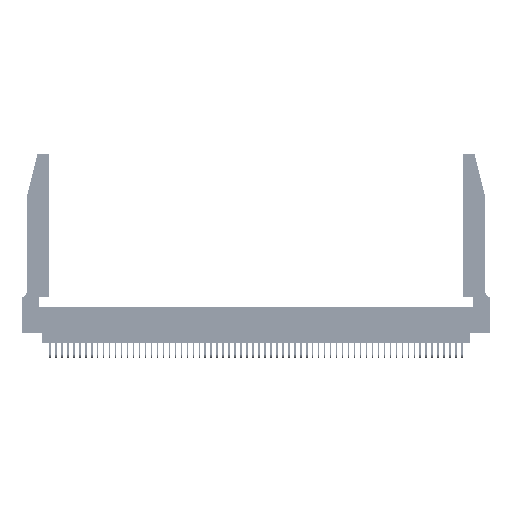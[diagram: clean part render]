
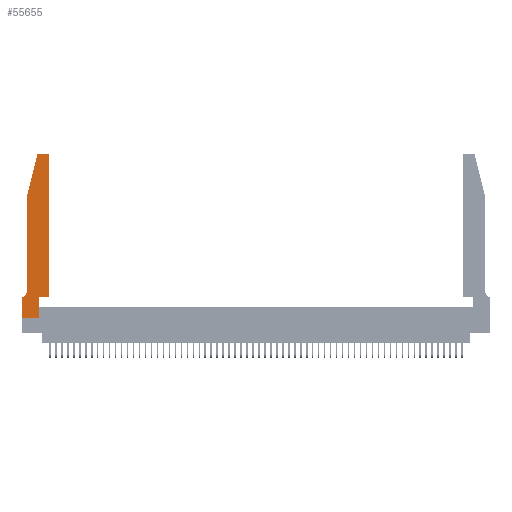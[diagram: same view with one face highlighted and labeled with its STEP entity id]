
A CAD part, top view. The second image highlights one B-rep face of the part: STEP entity #55655.
In plain terms, the highlighted planar face has unit normal (0, 0, 1).
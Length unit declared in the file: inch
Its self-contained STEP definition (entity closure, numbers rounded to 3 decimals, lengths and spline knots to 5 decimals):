
#858 = LINE ( 'NONE', #16642, #51080 ) ;
#1487 = VERTEX_POINT ( 'NONE', #41940 ) ;
#1556 = ORIENTED_EDGE ( 'NONE', *, *, #45499, .T. ) ;
#1739 = CARTESIAN_POINT ( 'NONE',  ( 0.2605, 2.75, 0.37 ) ) ;
#2333 = DIRECTION ( 'NONE',  ( 1., 0., 0. ) ) ;
#2833 = DIRECTION ( 'NONE',  ( 1., 0., 0. ) ) ;
#4481 = DIRECTION ( 'NONE',  ( 0., 0., 1. ) ) ;
#5484 = VERTEX_POINT ( 'NONE', #19264 ) ;
#6705 = CARTESIAN_POINT ( 'NONE',  ( 0.0755, 2., 0.37 ) ) ;
#7498 = ORIENTED_EDGE ( 'NONE', *, *, #34452, .T. ) ;
#7629 = VERTEX_POINT ( 'NONE', #12851 ) ;
#7697 = DIRECTION ( 'NONE',  ( 1., 0., 0. ) ) ;
#7972 = CARTESIAN_POINT ( 'NONE',  ( 0.0755, 0.35, 0.37 ) ) ;
#8842 = LINE ( 'NONE', #7972, #43009 ) ;
#9622 = CARTESIAN_POINT ( 'NONE',  ( 0.4205, 2.75, 0.37 ) ) ;
#10423 = AXIS2_PLACEMENT_3D ( 'NONE', #27438, #49858, #31884 ) ;
#10427 = AXIS2_PLACEMENT_3D ( 'NONE', #14665, #54387, #36827 ) ;
#10668 = AXIS2_PLACEMENT_3D ( 'NONE', #55692, #56073, #2333 ) ;
#10901 = FACE_OUTER_BOUND ( 'NONE', #43075, .T. ) ;
#11278 = DIRECTION ( 'NONE',  ( -1., 0., 0. ) ) ;
#11586 = DIRECTION ( 'NONE',  ( -0.239, -0.971, 0. ) ) ;
#11869 = CARTESIAN_POINT ( 'NONE',  ( 0.2865, 0.35, 0.37 ) ) ;
#12851 = CARTESIAN_POINT ( 'NONE',  ( 0.284, 2.75, 0.37 ) ) ;
#13425 = DIRECTION ( 'NONE',  ( 1., 0., 0. ) ) ;
#13940 = VECTOR ( 'NONE', #46292, 39.37008 ) ;
#14355 = ORIENTED_EDGE ( 'NONE', *, *, #27816, .T. ) ;
#14366 = LINE ( 'NONE', #51479, #42988 ) ;
#14377 = VECTOR ( 'NONE', #28451, 39.37008 ) ;
#14665 = CARTESIAN_POINT ( 'NONE',  ( 0.0055, 0.42, 0.37 ) ) ;
#14832 = CARTESIAN_POINT ( 'NONE',  ( 0.0755, 0.42, 0.37 ) ) ;
#16642 = CARTESIAN_POINT ( 'NONE',  ( 0., 0., 0.37 ) ) ;
#16815 = CARTESIAN_POINT ( 'NONE',  ( 0.4505, 0.35, 0.37 ) ) ;
#16957 = VERTEX_POINT ( 'NONE', #27746 ) ;
#17248 = ORIENTED_EDGE ( 'NONE', *, *, #18725, .T. ) ;
#18233 = EDGE_CURVE ( 'NONE', #22236, #16957, #29174, .T. ) ;
#18445 = EDGE_CURVE ( 'NONE', #31850, #26766, #36559, .T. ) ;
#18725 = EDGE_CURVE ( 'NONE', #16957, #31850, #8842, .T. ) ;
#18949 = LINE ( 'NONE', #29277, #37075 ) ;
#19264 = CARTESIAN_POINT ( 'NONE',  ( 0.25487, 2.72718, 0.37 ) ) ;
#20442 = VERTEX_POINT ( 'NONE', #11869 ) ;
#21576 = CARTESIAN_POINT ( 'NONE',  ( 0.4205, 2.72, 0.37 ) ) ;
#22236 = VERTEX_POINT ( 'NONE', #14832 ) ;
#22560 = CIRCLE ( 'NONE', #24779, 0.03 ) ;
#22872 = CARTESIAN_POINT ( 'NONE',  ( 0., 0., 0.37 ) ) ;
#24610 = VECTOR ( 'NONE', #11278, 39.37008 ) ;
#24753 = DIRECTION ( 'NONE',  ( 0., 1., 0. ) ) ;
#24779 = AXIS2_PLACEMENT_3D ( 'NONE', #21576, #4481, #13425 ) ;
#25440 = VERTEX_POINT ( 'NONE', #9622 ) ;
#25699 = EDGE_CURVE ( 'NONE', #1487, #20442, #14366, .T. ) ;
#26766 = VERTEX_POINT ( 'NONE', #22872 ) ;
#27021 = ORIENTED_EDGE ( 'NONE', *, *, #29974, .T. ) ;
#27438 = CARTESIAN_POINT ( 'NONE',  ( 0., 0.35, 0.37 ) ) ;
#27746 = CARTESIAN_POINT ( 'NONE',  ( 0.0055, 0.35, 0.37 ) ) ;
#27816 = EDGE_CURVE ( 'NONE', #28068, #25440, #22560, .T. ) ;
#28068 = VERTEX_POINT ( 'NONE', #37316 ) ;
#28074 = LINE ( 'NONE', #29671, #30833 ) ;
#28451 = DIRECTION ( 'NONE',  ( 0., -1., 0. ) ) ;
#28701 = CARTESIAN_POINT ( 'NONE',  ( 0.0755, 2., 0.37 ) ) ;
#29174 = CIRCLE ( 'NONE', #10427, 0.07 ) ;
#29277 = CARTESIAN_POINT ( 'NONE',  ( 0.0755, 2., 0.37 ) ) ;
#29671 = CARTESIAN_POINT ( 'NONE',  ( 0.4505, 0.35, 0.37 ) ) ;
#29974 = EDGE_CURVE ( 'NONE', #51574, #22236, #39682, .T. ) ;
#30833 = VECTOR ( 'NONE', #2833, 39.37008 ) ;
#31828 = CARTESIAN_POINT ( 'NONE',  ( 0., 0.35, 0.37 ) ) ;
#31850 = VERTEX_POINT ( 'NONE', #31828 ) ;
#31884 = DIRECTION ( 'NONE',  ( 1., 0., 0. ) ) ;
#31935 = CARTESIAN_POINT ( 'NONE',  ( 0.4505, 0.35, 0.37 ) ) ;
#32760 = CARTESIAN_POINT ( 'NONE',  ( 0., 0., 0.37 ) ) ;
#32862 = ORIENTED_EDGE ( 'NONE', *, *, #35316, .T. ) ;
#34040 = ORIENTED_EDGE ( 'NONE', *, *, #18445, .T. ) ;
#34452 = EDGE_CURVE ( 'NONE', #25440, #7629, #53190, .T. ) ;
#34831 = DIRECTION ( 'NONE',  ( -1., 0., 0. ) ) ;
#35316 = EDGE_CURVE ( 'NONE', #5484, #51574, #18949, .T. ) ;
#36559 = LINE ( 'NONE', #32760, #14377 ) ;
#36784 = LINE ( 'NONE', #31935, #43815 ) ;
#36827 = DIRECTION ( 'NONE',  ( -1., 0., 0. ) ) ;
#37075 = VECTOR ( 'NONE', #11586, 39.37008 ) ;
#37316 = CARTESIAN_POINT ( 'NONE',  ( 0.4505, 2.72, 0.37 ) ) ;
#38027 = EDGE_CURVE ( 'NONE', #20442, #43602, #28074, .T. ) ;
#38646 = EDGE_CURVE ( 'NONE', #26766, #1487, #858, .T. ) ;
#39682 = LINE ( 'NONE', #28701, #13940 ) ;
#39972 = EDGE_CURVE ( 'NONE', #7629, #5484, #48799, .T. ) ;
#41940 = CARTESIAN_POINT ( 'NONE',  ( 0.2865, 0., 0.37 ) ) ;
#42988 = VECTOR ( 'NONE', #24753, 39.37008 ) ;
#43009 = VECTOR ( 'NONE', #34831, 39.37008 ) ;
#43075 = EDGE_LOOP ( 'NONE', ( #7498, #53590, #32862, #27021, #45960, #17248, #34040, #44495, #45604, #52550, #1556, #14355 ) ) ;
#43602 = VERTEX_POINT ( 'NONE', #16815 ) ;
#43815 = VECTOR ( 'NONE', #45235, 39.37008 ) ;
#44495 = ORIENTED_EDGE ( 'NONE', *, *, #38646, .T. ) ;
#45235 = DIRECTION ( 'NONE',  ( 0., 1., 0. ) ) ;
#45499 = EDGE_CURVE ( 'NONE', #43602, #28068, #36784, .T. ) ;
#45604 = ORIENTED_EDGE ( 'NONE', *, *, #25699, .T. ) ;
#45960 = ORIENTED_EDGE ( 'NONE', *, *, #18233, .T. ) ;
#46292 = DIRECTION ( 'NONE',  ( 0., -1., 0. ) ) ;
#48799 = CIRCLE ( 'NONE', #10668, 0.03 ) ;
#49858 = DIRECTION ( 'NONE',  ( 0., 0., 1. ) ) ;
#51080 = VECTOR ( 'NONE', #7697, 39.37008 ) ;
#51479 = CARTESIAN_POINT ( 'NONE',  ( 0.2865, 0.35, 0.37 ) ) ;
#51574 = VERTEX_POINT ( 'NONE', #6705 ) ;
#52550 = ORIENTED_EDGE ( 'NONE', *, *, #38027, .T. ) ;
#53190 = LINE ( 'NONE', #1739, #24610 ) ;
#53590 = ORIENTED_EDGE ( 'NONE', *, *, #39972, .T. ) ;
#54121 = PLANE ( 'NONE',  #10423 ) ;
#54387 = DIRECTION ( 'NONE',  ( 0., 0., -1. ) ) ;
#55655 = ADVANCED_FACE ( 'NONE', ( #10901 ), #54121, .T. ) ;
#55692 = CARTESIAN_POINT ( 'NONE',  ( 0.284, 2.72, 0.37 ) ) ;
#56073 = DIRECTION ( 'NONE',  ( 0., 0., 1. ) ) ;
